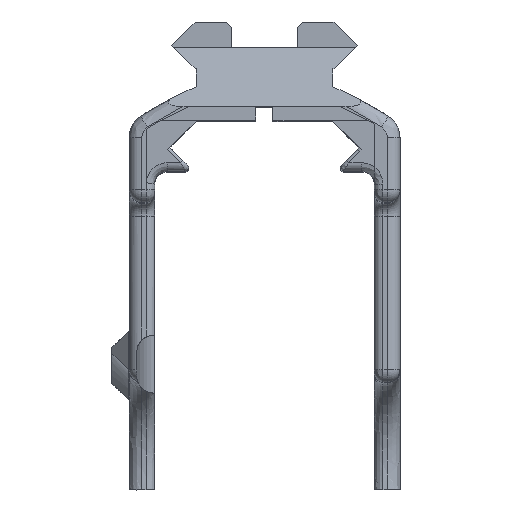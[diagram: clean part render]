
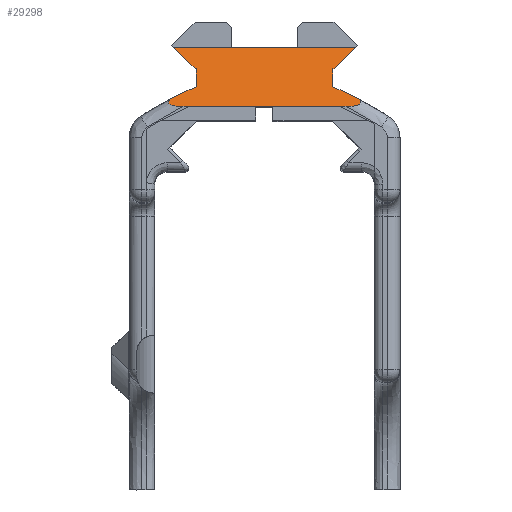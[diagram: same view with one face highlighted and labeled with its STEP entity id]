
A CAD part, left-side view. The second image highlights one B-rep face of the part: STEP entity #29298.
In plain terms, the highlighted planar face has unit normal (-0.616, 0, 0.788).
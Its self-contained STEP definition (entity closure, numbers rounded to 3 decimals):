
#721=B_SPLINE_CURVE_WITH_KNOTS('',3,(#55801,#55802,#55803,#55804,#55805,
#55806,#55807,#55808,#55809,#55810,#55811,#55812,#55813,#55814,#55815,#55816),
 .UNSPECIFIED.,.F.,.F.,(4,2,2,2,2,2,2,4),(-0.456,-0.303,
-0.249,-0.214,-0.183,-0.147,
-0.091,0.),.UNSPECIFIED.);
#722=B_SPLINE_CURVE_WITH_KNOTS('',3,(#55818,#55819,#55820,#55821),
 .UNSPECIFIED.,.F.,.F.,(4,4),(-1.173,-0.856),
 .UNSPECIFIED.);
#723=B_SPLINE_CURVE_WITH_KNOTS('',3,(#55837,#55838,#55839,#55840,#55841,
#55842,#55843),.UNSPECIFIED.,.F.,.F.,(4,3,4),(0.,0.177,0.315),
 .UNSPECIFIED.);
#724=B_SPLINE_CURVE_WITH_KNOTS('',3,(#55845,#55846,#55847,#55848,#55849,
#55850,#55851,#55852,#55853,#55854,#55855,#55856,#55857,#55858,#55859,#55860),
 .UNSPECIFIED.,.F.,.F.,(4,2,2,2,2,2,2,4),(-0.293,-0.237,
-0.203,-0.181,-0.161,-0.138,
-0.102,0.),.UNSPECIFIED.);
#1146=PLANE('',#29812);
#2625=FACE_OUTER_BOUND('',#4238,.T.);
#4238=EDGE_LOOP('',(#24724,#24725,#24726,#24727,#24728,#24729,#24730,#24731,
#24732,#24733,#24734,#24735,#24736,#24737));
#5856=LINE('',#55799,#7872);
#5857=LINE('',#55823,#7873);
#5858=LINE('',#55825,#7874);
#5859=LINE('',#55827,#7875);
#5860=LINE('',#55829,#7876);
#5861=LINE('',#55831,#7877);
#5862=LINE('',#55833,#7878);
#5863=LINE('',#55835,#7879);
#5864=LINE('',#55862,#7880);
#5865=LINE('',#55863,#7881);
#7872=VECTOR('',#31677,10.);
#7873=VECTOR('',#31678,10.);
#7874=VECTOR('',#31679,10.);
#7875=VECTOR('',#31680,10.);
#7876=VECTOR('',#31681,10.);
#7877=VECTOR('',#31682,10.);
#7878=VECTOR('',#31683,10.);
#7879=VECTOR('',#31684,10.);
#7880=VECTOR('',#31685,10.);
#7881=VECTOR('',#31686,10.);
#12671=VERTEX_POINT('',#55797);
#12672=VERTEX_POINT('',#55798);
#12673=VERTEX_POINT('',#55800);
#12674=VERTEX_POINT('',#55817);
#12675=VERTEX_POINT('',#55822);
#12676=VERTEX_POINT('',#55824);
#12677=VERTEX_POINT('',#55826);
#12678=VERTEX_POINT('',#55828);
#12679=VERTEX_POINT('',#55830);
#12680=VERTEX_POINT('',#55832);
#12681=VERTEX_POINT('',#55834);
#12682=VERTEX_POINT('',#55836);
#12683=VERTEX_POINT('',#55844);
#12684=VERTEX_POINT('',#55861);
#16813=EDGE_CURVE('',#12671,#12672,#5856,.T.);
#16814=EDGE_CURVE('',#12672,#12673,#721,.T.);
#16815=EDGE_CURVE('',#12673,#12674,#722,.T.);
#16816=EDGE_CURVE('',#12675,#12674,#5857,.T.);
#16817=EDGE_CURVE('',#12676,#12675,#5858,.T.);
#16818=EDGE_CURVE('',#12677,#12676,#5859,.T.);
#16819=EDGE_CURVE('',#12678,#12677,#5860,.T.);
#16820=EDGE_CURVE('',#12679,#12678,#5861,.T.);
#16821=EDGE_CURVE('',#12680,#12679,#5862,.T.);
#16822=EDGE_CURVE('',#12681,#12680,#5863,.T.);
#16823=EDGE_CURVE('',#12682,#12681,#723,.T.);
#16824=EDGE_CURVE('',#12682,#12683,#724,.T.);
#16825=EDGE_CURVE('',#12683,#12684,#5864,.T.);
#16826=EDGE_CURVE('',#12684,#12671,#5865,.T.);
#24724=ORIENTED_EDGE('',*,*,#16813,.T.);
#24725=ORIENTED_EDGE('',*,*,#16814,.T.);
#24726=ORIENTED_EDGE('',*,*,#16815,.T.);
#24727=ORIENTED_EDGE('',*,*,#16816,.F.);
#24728=ORIENTED_EDGE('',*,*,#16817,.F.);
#24729=ORIENTED_EDGE('',*,*,#16818,.F.);
#24730=ORIENTED_EDGE('',*,*,#16819,.F.);
#24731=ORIENTED_EDGE('',*,*,#16820,.F.);
#24732=ORIENTED_EDGE('',*,*,#16821,.F.);
#24733=ORIENTED_EDGE('',*,*,#16822,.F.);
#24734=ORIENTED_EDGE('',*,*,#16823,.F.);
#24735=ORIENTED_EDGE('',*,*,#16824,.T.);
#24736=ORIENTED_EDGE('',*,*,#16825,.T.);
#24737=ORIENTED_EDGE('',*,*,#16826,.T.);
#29298=ADVANCED_FACE('',(#2625),#1146,.T.);
#29812=AXIS2_PLACEMENT_3D('',#55796,#31675,#31676);
#31675=DIRECTION('center_axis',(-0.616,0.,
0.788));
#31676=DIRECTION('ref_axis',(0.788,0.,0.616));
#31677=DIRECTION('',(0.,-1.,0.));
#31678=DIRECTION('',(-0.788,0.,-0.616));
#31679=DIRECTION('',(0.,1.,0.));
#31680=DIRECTION('',(-0.671,0.524,-0.524));
#31681=DIRECTION('',(0.,-1.,0.));
#31682=DIRECTION('',(0.671,0.524,0.524));
#31683=DIRECTION('',(0.,1.,0.));
#31684=DIRECTION('',(0.788,0.,0.616));
#31685=DIRECTION('',(0.,-1.,0.));
#31686=DIRECTION('',(0.,-1.,0.));
#55796=CARTESIAN_POINT('Origin',(2806.441,450.735,177.416));
#55797=CARTESIAN_POINT('',(2737.227,441.964,123.34));
#55798=CARTESIAN_POINT('',(2737.227,441.162,123.34));
#55799=CARTESIAN_POINT('',(2737.227,444.284,123.34));
#55800=CARTESIAN_POINT('',(2738.729,440.156,124.513));
#55801=CARTESIAN_POINT('Ctrl Pts',(2737.227,441.162,123.34));
#55802=CARTESIAN_POINT('Ctrl Pts',(2737.227,440.83,123.34));
#55803=CARTESIAN_POINT('Ctrl Pts',(2737.248,440.405,123.356));
#55804=CARTESIAN_POINT('Ctrl Pts',(2737.378,439.934,123.458));
#55805=CARTESIAN_POINT('Ctrl Pts',(2737.423,439.812,123.493));
#55806=CARTESIAN_POINT('Ctrl Pts',(2737.525,439.642,123.572));
#55807=CARTESIAN_POINT('Ctrl Pts',(2737.572,439.583,123.609));
#55808=CARTESIAN_POINT('Ctrl Pts',(2737.677,439.497,123.691));
#55809=CARTESIAN_POINT('Ctrl Pts',(2737.731,439.469,123.733));
#55810=CARTESIAN_POINT('Ctrl Pts',(2737.856,439.439,123.831));
#55811=CARTESIAN_POINT('Ctrl Pts',(2737.924,439.443,123.884));
#55812=CARTESIAN_POINT('Ctrl Pts',(2738.093,439.489,124.016));
#55813=CARTESIAN_POINT('Ctrl Pts',(2738.192,439.549,124.094));
#55814=CARTESIAN_POINT('Ctrl Pts',(2738.427,439.741,124.277));
#55815=CARTESIAN_POINT('Ctrl Pts',(2738.578,439.92,124.395));
#55816=CARTESIAN_POINT('Ctrl Pts',(2738.729,440.156,124.513));
#55817=CARTESIAN_POINT('',(2740.2,442.734,125.663));
#55818=CARTESIAN_POINT('Ctrl Pts',(2738.729,440.156,124.513));
#55819=CARTESIAN_POINT('Ctrl Pts',(2739.251,440.971,124.921));
#55820=CARTESIAN_POINT('Ctrl Pts',(2739.751,441.833,125.311));
#55821=CARTESIAN_POINT('Ctrl Pts',(2740.2,442.734,125.663));
#55822=CARTESIAN_POINT('',(2742.894,442.734,127.767));
#55823=CARTESIAN_POINT('',(2740.026,442.734,125.527));
#55824=CARTESIAN_POINT('',(2742.894,442.581,127.767));
#55825=CARTESIAN_POINT('',(2742.894,446.908,127.767));
#55826=CARTESIAN_POINT('',(2746.08,440.092,130.256));
#55827=CARTESIAN_POINT('',(2740.257,444.641,125.707));
#55828=CARTESIAN_POINT('',(2746.08,461.377,130.256));
#55829=CARTESIAN_POINT('',(2746.08,452.916,130.256));
#55830=CARTESIAN_POINT('',(2742.894,458.888,127.767));
#55831=CARTESIAN_POINT('',(2739.468,456.211,125.091));
#55832=CARTESIAN_POINT('',(2742.894,458.734,127.767));
#55833=CARTESIAN_POINT('',(2742.894,454.984,127.767));
#55834=CARTESIAN_POINT('',(2740.2,458.734,125.662));
#55835=CARTESIAN_POINT('',(2738.572,458.734,124.39));
#55836=CARTESIAN_POINT('',(2738.729,461.312,124.513));
#55837=CARTESIAN_POINT('Ctrl Pts',(2738.729,461.312,124.513));
#55838=CARTESIAN_POINT('Ctrl Pts',(2739.022,460.855,124.742));
#55839=CARTESIAN_POINT('Ctrl Pts',(2739.307,460.384,124.965));
#55840=CARTESIAN_POINT('Ctrl Pts',(2739.58,459.9,125.178));
#55841=CARTESIAN_POINT('Ctrl Pts',(2739.795,459.519,125.346));
#55842=CARTESIAN_POINT('Ctrl Pts',(2740.002,459.131,125.508));
#55843=CARTESIAN_POINT('Ctrl Pts',(2740.2,458.734,125.662));
#55844=CARTESIAN_POINT('',(2737.227,460.306,123.34));
#55845=CARTESIAN_POINT('Ctrl Pts',(2738.729,461.312,124.513));
#55846=CARTESIAN_POINT('Ctrl Pts',(2738.588,461.532,124.403));
#55847=CARTESIAN_POINT('Ctrl Pts',(2738.447,461.702,124.293));
#55848=CARTESIAN_POINT('Ctrl Pts',(2738.227,461.893,124.121));
#55849=CARTESIAN_POINT('Ctrl Pts',(2738.135,461.956,124.049));
#55850=CARTESIAN_POINT('Ctrl Pts',(2737.975,462.015,123.924));
#55851=CARTESIAN_POINT('Ctrl Pts',(2737.909,462.027,123.872));
#55852=CARTESIAN_POINT('Ctrl Pts',(2737.784,462.016,123.775));
#55853=CARTESIAN_POINT('Ctrl Pts',(2737.728,461.997,123.731));
#55854=CARTESIAN_POINT('Ctrl Pts',(2737.614,461.926,123.642));
#55855=CARTESIAN_POINT('Ctrl Pts',(2737.561,461.872,123.601));
#55856=CARTESIAN_POINT('Ctrl Pts',(2737.446,461.706,123.511));
#55857=CARTESIAN_POINT('Ctrl Pts',(2737.395,461.582,123.471));
#55858=CARTESIAN_POINT('Ctrl Pts',(2737.25,461.097,123.357));
#55859=CARTESIAN_POINT('Ctrl Pts',(2737.227,460.646,123.34));
#55860=CARTESIAN_POINT('Ctrl Pts',(2737.227,460.306,123.34));
#55861=CARTESIAN_POINT('',(2737.227,459.503,123.34));
#55862=CARTESIAN_POINT('',(2737.227,444.284,123.34));
#55863=CARTESIAN_POINT('',(2737.227,457.367,123.34));
